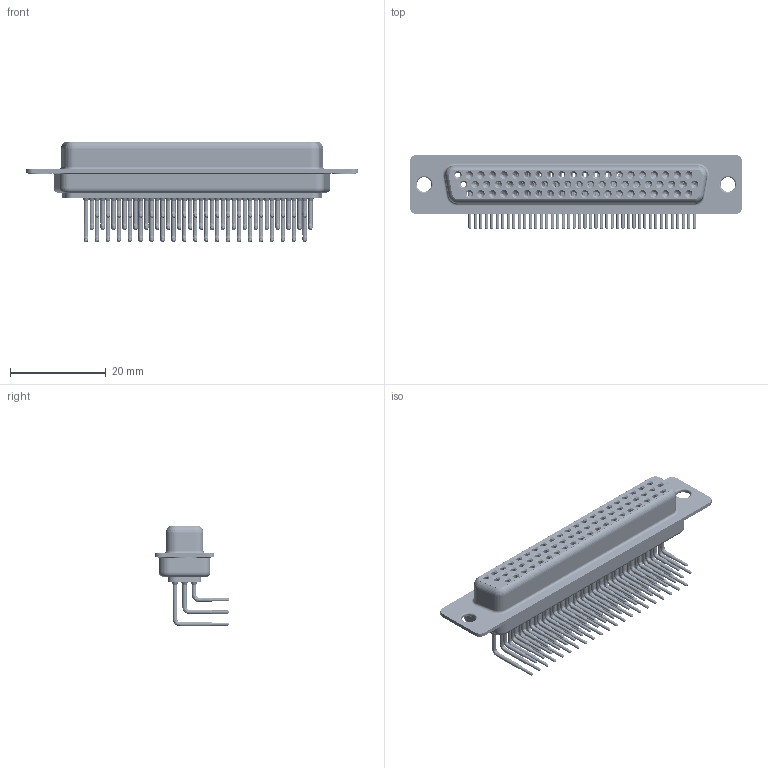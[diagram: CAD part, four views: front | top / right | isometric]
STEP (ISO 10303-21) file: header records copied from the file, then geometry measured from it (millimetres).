
FILE_DESCRIPTION (( 'STEP AP203' ), '1' );
FILE_NAME ('634-M62-263-WT1.STEP', '2018-09-28T02:52:36', ( '' ), ( '' ), 'SwSTEP 2.0', 'SolidWorks 2016', '' );
FILE_SCHEMA (( 'CONFIG_CONTROL_DESIGN' ));
Length unit declared in the file: millimetre
Products named in the file (8): 634M Shell Front_62 Contacts; 634M Shell Rear_62 Contacts; 634M Contact Row 1; 634M Contact Row 2; 634M Contact Row 3; 634M Thru Hole Rivet; 634-M62-263-WT1; 634M Housing_62 Contacts
Assembly tree (67 placements, depth 2):
  634-M62-263-WT1
    634M Housing_62 Contacts
    634M Shell Front_62 Contacts
    634M Shell Rear_62 Contacts
    634M Contact Row 1  x21
    634M Contact Row 2  x21
    634M Contact Row 3  x20
    634M Thru Hole Rivet  x2
Bounding box: 69.4 x 15.6 x 21.02 mm (x, y, z)
Volume: 5325.8 mm3; surface area: 17717.4 mm2
Topology: 67 solids, 67 shells, 3539 faces, 8973 edges, 5641 vertices
Faces by surface type: cylinder 1547, plane 997, cone 682, bspline 248, torus 65
Entity records: 36144 total; most frequent: DIRECTION 6531, CARTESIAN_POINT 5937, ORIENTED_EDGE 5216, AXIS2_PLACEMENT_3D 2775, EDGE_CURVE 2608, VERTEX_POINT 1664, CIRCLE 1558, EDGE_LOOP 1498
